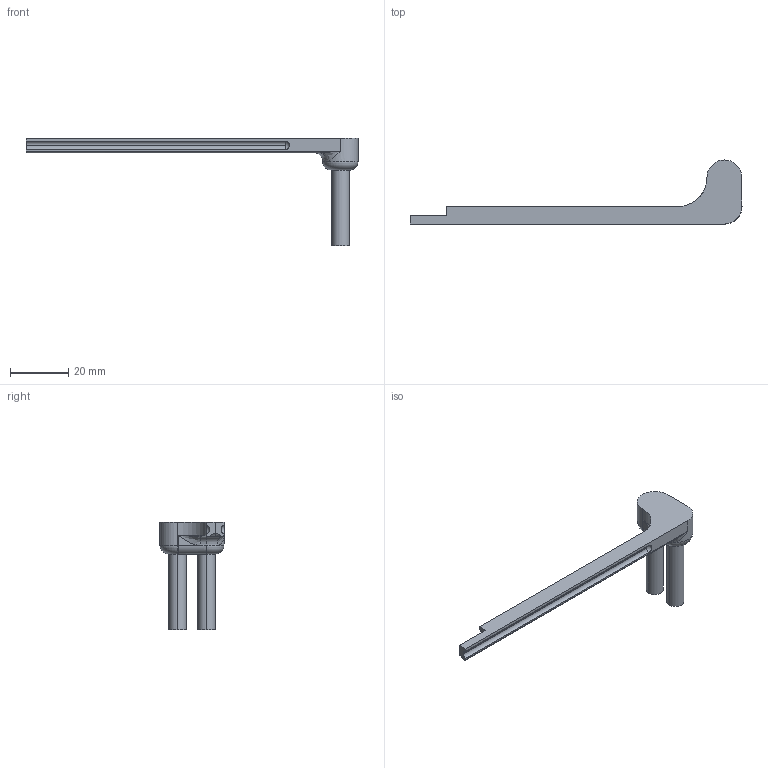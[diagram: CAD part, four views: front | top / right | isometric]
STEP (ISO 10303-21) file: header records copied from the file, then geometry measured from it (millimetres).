
FILE_DESCRIPTION (( 'STEP AP214' ), '1' );
FILE_NAME ('Trigger_Rod_Right_1.step', '2014-05-14T06:09:29', ( 'WarFairy' ), ( '' ), 'SwSTEP 2.0', 'SolidWorks 2013', '' );
FILE_SCHEMA (( 'AUTOMOTIVE_DESIGN' ));
Length unit declared in the file: inch
Products named in the file (1): Trigger_Rod_Right_1
Bounding box: 114.3 x 22.07 x 37.1 mm (x, y, z)
Volume: 6363.1 mm3; surface area: 4368.8 mm2
Topology: 1 solids, 1 shells, 49 faces, 121 edges, 74 vertices
Faces by surface type: cylinder 20, plane 16, torus 11, bspline 2
Entity records: 1801 total; most frequent: CARTESIAN_POINT 593, DIRECTION 257, ORIENTED_EDGE 240, EDGE_CURVE 120, AXIS2_PLACEMENT_3D 100, VERTEX_POINT 74, LINE 57, VECTOR 57
